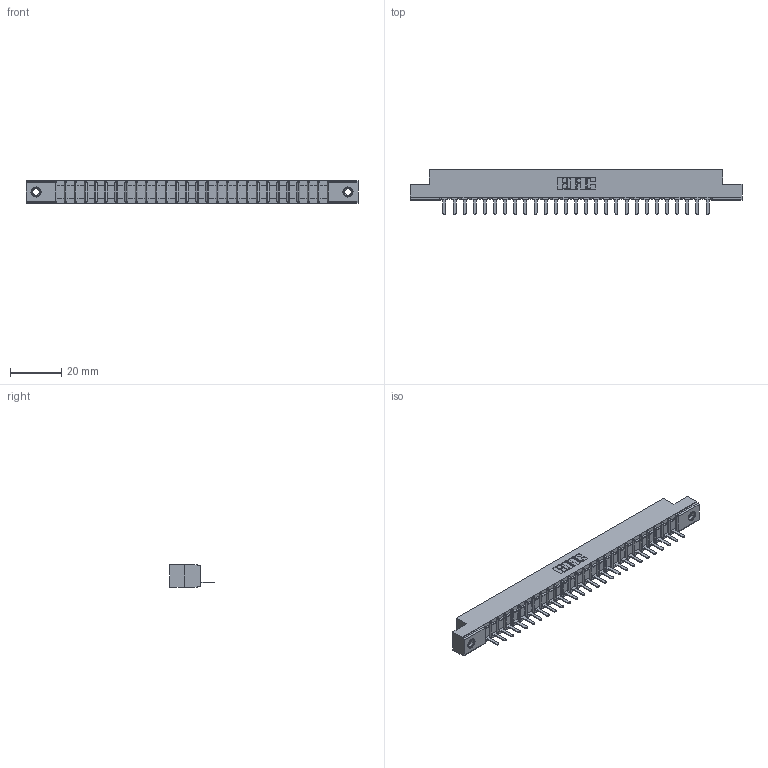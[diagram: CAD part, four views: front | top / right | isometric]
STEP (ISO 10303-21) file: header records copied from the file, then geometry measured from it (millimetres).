
FILE_DESCRIPTION (( 'STEP AP203' ), '1' );
FILE_NAME ('357-027-521-107.STEP', '2018-08-09T04:52:02', ( '' ), ( '' ), 'SwSTEP 2.0', 'SolidWorks 2016', '' );
FILE_SCHEMA (( 'CONFIG_CONTROL_DESIGN' ));
Length unit declared in the file: inch
Products named in the file (4): 307 Part_.156 Dia Mounting Holes; 307-290-002_521; 345-250-001_345-250-005-103; 357-027-521-107
Assembly tree (30 placements, depth 2):
  357-027-521-107
    307 Part_.156 Dia Mounting Holes
    307-290-002_521  x27
    345-250-001_345-250-005-103  x2
Bounding box: 130 x 17.42 x 8.71 mm (x, y, z)
Volume: 8572.8 mm3; surface area: 15922.3 mm2
Topology: 30 solids, 30 shells, 2204 faces, 6723 edges, 4398 vertices
Faces by surface type: plane 1317, cylinder 815, sphere 56, cone 12, torus 4
Entity records: 26899 total; most frequent: CARTESIAN_POINT 4515, ORIENTED_EDGE 4498, DIRECTION 4403, EDGE_CURVE 2249, LINE 1715, VECTOR 1715, VERTEX_POINT 1456, AXIS2_PLACEMENT_3D 1344
